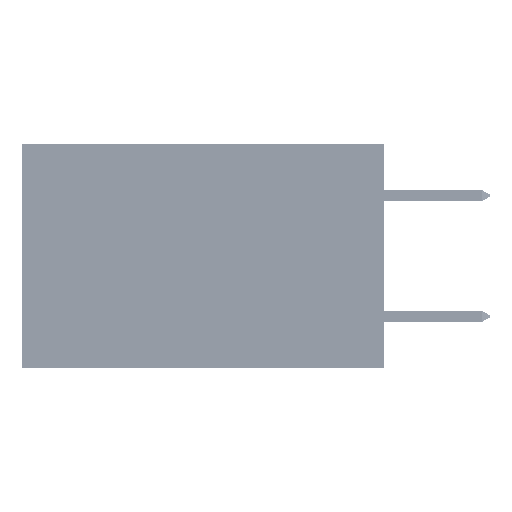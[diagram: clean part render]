
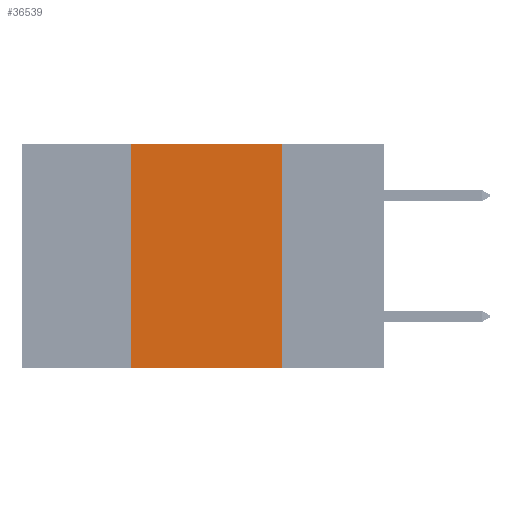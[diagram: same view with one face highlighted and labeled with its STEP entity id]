
A CAD part, left-side view. The second image highlights one B-rep face of the part: STEP entity #36539.
In plain terms, the highlighted planar face has unit normal (-1, 0, 0).
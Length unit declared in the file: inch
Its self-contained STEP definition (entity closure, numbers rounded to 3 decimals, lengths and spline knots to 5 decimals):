
#1481 = DIRECTION ( 'NONE',  ( 0., 0., -1. ) ) ;
#2633 = CARTESIAN_POINT ( 'NONE',  ( 0., 0.42, 0. ) ) ;
#3499 = ORIENTED_EDGE ( 'NONE', *, *, #38871, .F. ) ;
#3777 = ORIENTED_EDGE ( 'NONE', *, *, #24628, .F. ) ;
#4932 = CARTESIAN_POINT ( 'NONE',  ( 0., 0.6, 0. ) ) ;
#8126 = VECTOR ( 'NONE', #1481, 39.37008 ) ;
#8399 = FACE_OUTER_BOUND ( 'NONE', #22165, .T. ) ;
#12856 = VERTEX_POINT ( 'NONE', #32432 ) ;
#13047 = CARTESIAN_POINT ( 'NONE',  ( 0., 0.42, 0. ) ) ;
#13337 = LINE ( 'NONE', #40513, #28572 ) ;
#13751 = CARTESIAN_POINT ( 'NONE',  ( 0., 0.6, 0. ) ) ;
#14188 = ORIENTED_EDGE ( 'NONE', *, *, #43232, .F. ) ;
#15706 = LINE ( 'NONE', #42874, #8126 ) ;
#18859 = VERTEX_POINT ( 'NONE', #27370 ) ;
#19606 = EDGE_CURVE ( 'NONE', #12856, #18859, #13337, .T. ) ;
#19618 = DIRECTION ( 'NONE',  ( 1., 0., 0. ) ) ;
#20076 = VECTOR ( 'NONE', #28234, 39.37008 ) ;
#21449 = LINE ( 'NONE', #13751, #29886 ) ;
#22085 = VERTEX_POINT ( 'NONE', #32358 ) ;
#22165 = EDGE_LOOP ( 'NONE', ( #3777, #14188, #3499, #33674 ) ) ;
#23837 = PLANE ( 'NONE',  #48605 ) ;
#24628 = EDGE_CURVE ( 'NONE', #22085, #18859, #15706, .T. ) ;
#26101 = VERTEX_POINT ( 'NONE', #2633 ) ;
#27370 = CARTESIAN_POINT ( 'NONE',  ( 0., 0.17, -0.37 ) ) ;
#28234 = DIRECTION ( 'NONE',  ( 0., 0., 1. ) ) ;
#28572 = VECTOR ( 'NONE', #44251, 39.37008 ) ;
#28680 = DIRECTION ( 'NONE',  ( 0., -1., 0. ) ) ;
#29886 = VECTOR ( 'NONE', #28680, 39.37008 ) ;
#32358 = CARTESIAN_POINT ( 'NONE',  ( 0., 0.17, 0. ) ) ;
#32432 = CARTESIAN_POINT ( 'NONE',  ( 0., 0.42, -0.37 ) ) ;
#33674 = ORIENTED_EDGE ( 'NONE', *, *, #19606, .T. ) ;
#35309 = DIRECTION ( 'NONE',  ( 0., 0., -1. ) ) ;
#36206 = LINE ( 'NONE', #13047, #20076 ) ;
#36539 = ADVANCED_FACE ( 'NONE', ( #8399 ), #23837, .F. ) ;
#38871 = EDGE_CURVE ( 'NONE', #12856, #26101, #36206, .T. ) ;
#40513 = CARTESIAN_POINT ( 'NONE',  ( 0., 0.6, -0.37 ) ) ;
#42874 = CARTESIAN_POINT ( 'NONE',  ( 0., 0.17, 0. ) ) ;
#43232 = EDGE_CURVE ( 'NONE', #26101, #22085, #21449, .T. ) ;
#44251 = DIRECTION ( 'NONE',  ( 0., -1., 0. ) ) ;
#48605 = AXIS2_PLACEMENT_3D ( 'NONE', #4932, #19618, #35309 ) ;
